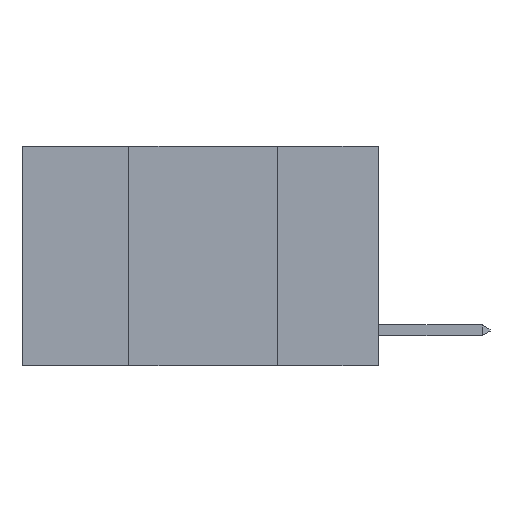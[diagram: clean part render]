
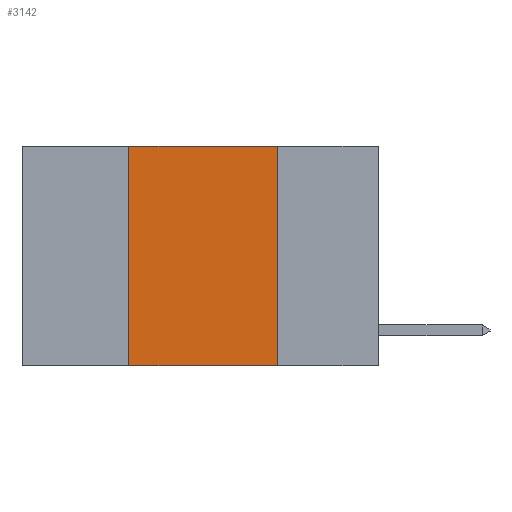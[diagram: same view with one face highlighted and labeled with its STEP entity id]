
A CAD part, left-side view. The second image highlights one B-rep face of the part: STEP entity #3142.
In plain terms, the highlighted planar face has unit normal (-1, 0, 0).
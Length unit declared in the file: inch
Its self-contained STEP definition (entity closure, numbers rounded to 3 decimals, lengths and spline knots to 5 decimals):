
#226 = VERTEX_POINT ( 'NONE', #7103 ) ;
#597 = CARTESIAN_POINT ( 'NONE',  ( 0., 0.42, 0. ) ) ;
#852 = DIRECTION ( 'NONE',  ( 0., 0., -1. ) ) ;
#1270 = VECTOR ( 'NONE', #9765, 39.37008 ) ;
#1479 = DIRECTION ( 'NONE',  ( 0., 0., 1. ) ) ;
#1700 = CARTESIAN_POINT ( 'NONE',  ( 0., 0.42, 0. ) ) ;
#3128 = VERTEX_POINT ( 'NONE', #1700 ) ;
#3142 = ADVANCED_FACE ( 'NONE', ( #3963 ), #9327, .F. ) ;
#3652 = LINE ( 'NONE', #8108, #1270 ) ;
#3815 = LINE ( 'NONE', #4215, #7971 ) ;
#3963 = FACE_OUTER_BOUND ( 'NONE', #9985, .T. ) ;
#4215 = CARTESIAN_POINT ( 'NONE',  ( 0., 0.17, 0. ) ) ;
#4237 = EDGE_CURVE ( 'NONE', #4473, #10660, #3815, .T. ) ;
#4473 = VERTEX_POINT ( 'NONE', #7833 ) ;
#4549 = VECTOR ( 'NONE', #9814, 39.37008 ) ;
#4786 = EDGE_CURVE ( 'NONE', #226, #3128, #5231, .T. ) ;
#4858 = CARTESIAN_POINT ( 'NONE',  ( 0., 0.6, 0. ) ) ;
#5231 = LINE ( 'NONE', #597, #9120 ) ;
#5344 = EDGE_CURVE ( 'NONE', #226, #10660, #3652, .T. ) ;
#6035 = DIRECTION ( 'NONE',  ( 1., 0., 0. ) ) ;
#6092 = AXIS2_PLACEMENT_3D ( 'NONE', #10962, #6035, #852 ) ;
#7014 = LINE ( 'NONE', #4858, #4549 ) ;
#7103 = CARTESIAN_POINT ( 'NONE',  ( 0., 0.42, -0.37 ) ) ;
#7642 = CARTESIAN_POINT ( 'NONE',  ( 0., 0.17, -0.37 ) ) ;
#7833 = CARTESIAN_POINT ( 'NONE',  ( 0., 0.17, 0. ) ) ;
#7971 = VECTOR ( 'NONE', #9171, 39.37008 ) ;
#8108 = CARTESIAN_POINT ( 'NONE',  ( 0., 0.6, -0.37 ) ) ;
#8509 = ORIENTED_EDGE ( 'NONE', *, *, #4237, .F. ) ;
#8540 = ORIENTED_EDGE ( 'NONE', *, *, #10522, .F. ) ;
#8770 = ORIENTED_EDGE ( 'NONE', *, *, #4786, .F. ) ;
#8780 = ORIENTED_EDGE ( 'NONE', *, *, #5344, .T. ) ;
#9120 = VECTOR ( 'NONE', #1479, 39.37008 ) ;
#9171 = DIRECTION ( 'NONE',  ( 0., 0., -1. ) ) ;
#9327 = PLANE ( 'NONE',  #6092 ) ;
#9765 = DIRECTION ( 'NONE',  ( 0., -1., 0. ) ) ;
#9814 = DIRECTION ( 'NONE',  ( 0., -1., 0. ) ) ;
#9985 = EDGE_LOOP ( 'NONE', ( #8509, #8540, #8770, #8780 ) ) ;
#10522 = EDGE_CURVE ( 'NONE', #3128, #4473, #7014, .T. ) ;
#10660 = VERTEX_POINT ( 'NONE', #7642 ) ;
#10962 = CARTESIAN_POINT ( 'NONE',  ( 0., 0.6, 0. ) ) ;
